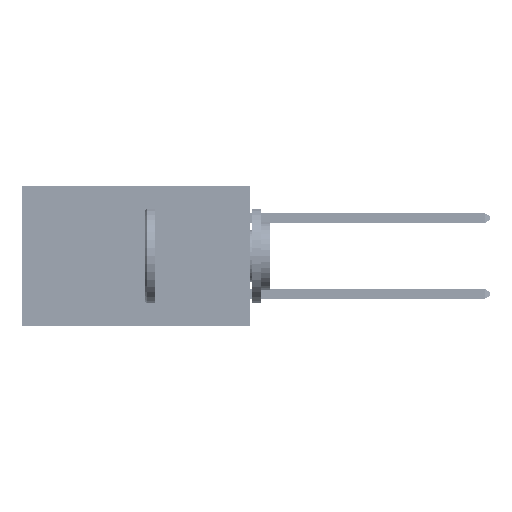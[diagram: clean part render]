
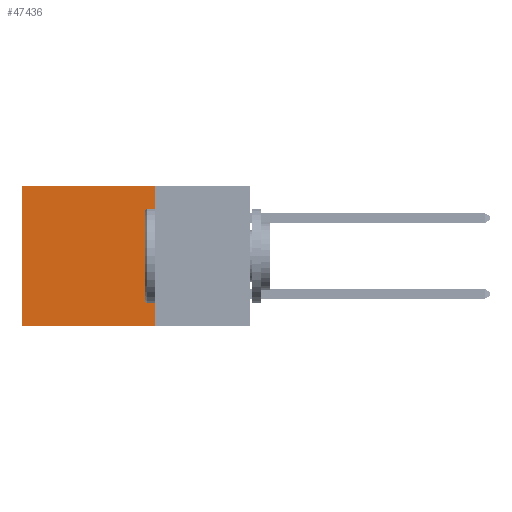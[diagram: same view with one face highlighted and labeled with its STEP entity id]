
A CAD part, left-side view. The second image highlights one B-rep face of the part: STEP entity #47436.
In plain terms, the highlighted planar face has unit normal (-1, 0, 0).
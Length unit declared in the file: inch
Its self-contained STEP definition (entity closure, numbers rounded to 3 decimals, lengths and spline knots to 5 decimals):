
#157 = DIRECTION ( 'NONE',  ( 0., 1., 0. ) ) ;
#176 = EDGE_CURVE ( 'NONE', #20249, #36498, #25073, .T. ) ;
#868 = AXIS2_PLACEMENT_3D ( 'NONE', #7421, #7256, #48261 ) ;
#2560 = ORIENTED_EDGE ( 'NONE', *, *, #176, .T. ) ;
#2584 = DIRECTION ( 'NONE',  ( 0., 1., 0. ) ) ;
#4113 = ORIENTED_EDGE ( 'NONE', *, *, #45465, .T. ) ;
#4659 = VECTOR ( 'NONE', #2584, 39.37008 ) ;
#6309 = CARTESIAN_POINT ( 'NONE',  ( 0.2875, 0.25, -0.37 ) ) ;
#7192 = VERTEX_POINT ( 'NONE', #33280 ) ;
#7256 = DIRECTION ( 'NONE',  ( 1., 0., 0. ) ) ;
#7421 = CARTESIAN_POINT ( 'NONE',  ( 0.2875, 0.25, 0. ) ) ;
#7611 = CARTESIAN_POINT ( 'NONE',  ( 0.2875, 0.6, 0. ) ) ;
#8259 = FACE_OUTER_BOUND ( 'NONE', #12087, .T. ) ;
#12087 = EDGE_LOOP ( 'NONE', ( #4113, #30747, #23762, #2560 ) ) ;
#19211 = DIRECTION ( 'NONE',  ( 0., 0., -1. ) ) ;
#20249 = VERTEX_POINT ( 'NONE', #48058 ) ;
#23762 = ORIENTED_EDGE ( 'NONE', *, *, #44200, .F. ) ;
#24245 = DIRECTION ( 'NONE',  ( 0., 0., -1. ) ) ;
#25073 = LINE ( 'NONE', #32603, #52344 ) ;
#27384 = CARTESIAN_POINT ( 'NONE',  ( 0.2875, 0.25, 0. ) ) ;
#30747 = ORIENTED_EDGE ( 'NONE', *, *, #33552, .F. ) ;
#32603 = CARTESIAN_POINT ( 'NONE',  ( 0.2875, 0.25, 0. ) ) ;
#33280 = CARTESIAN_POINT ( 'NONE',  ( 0.2875, 0.25, -0.37 ) ) ;
#33552 = EDGE_CURVE ( 'NONE', #7192, #39835, #47229, .T. ) ;
#35168 = LINE ( 'NONE', #51402, #47246 ) ;
#36498 = VERTEX_POINT ( 'NONE', #7611 ) ;
#39835 = VERTEX_POINT ( 'NONE', #44979 ) ;
#44170 = PLANE ( 'NONE',  #868 ) ;
#44200 = EDGE_CURVE ( 'NONE', #20249, #7192, #46731, .T. ) ;
#44979 = CARTESIAN_POINT ( 'NONE',  ( 0.2875, 0.6, -0.37 ) ) ;
#45451 = VECTOR ( 'NONE', #19211, 39.37008 ) ;
#45465 = EDGE_CURVE ( 'NONE', #36498, #39835, #35168, .T. ) ;
#46731 = LINE ( 'NONE', #27384, #45451 ) ;
#47229 = LINE ( 'NONE', #6309, #4659 ) ;
#47246 = VECTOR ( 'NONE', #24245, 39.37008 ) ;
#47436 = ADVANCED_FACE ( 'NONE', ( #8259 ), #44170, .F. ) ;
#48058 = CARTESIAN_POINT ( 'NONE',  ( 0.2875, 0.25, 0. ) ) ;
#48261 = DIRECTION ( 'NONE',  ( 0., 0., -1. ) ) ;
#51402 = CARTESIAN_POINT ( 'NONE',  ( 0.2875, 0.6, 0. ) ) ;
#52344 = VECTOR ( 'NONE', #157, 39.37008 ) ;
